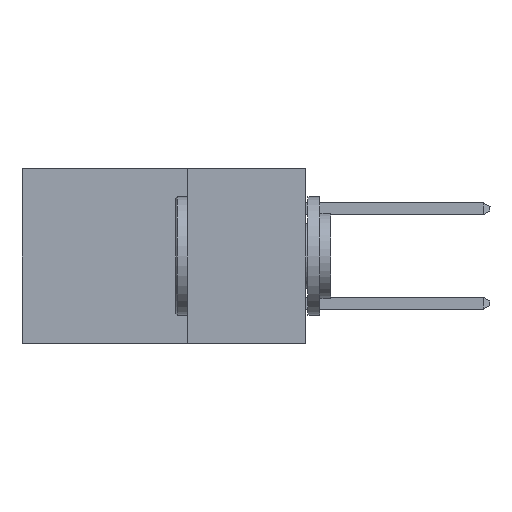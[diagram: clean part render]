
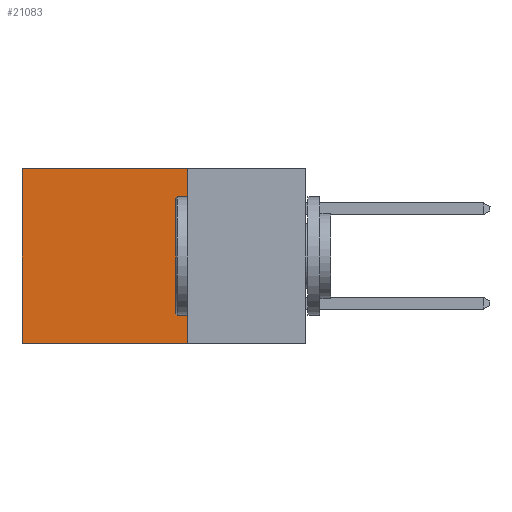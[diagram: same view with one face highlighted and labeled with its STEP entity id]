
A CAD part, left-side view. The second image highlights one B-rep face of the part: STEP entity #21083.
In plain terms, the highlighted planar face has unit normal (-1, 0, 0).
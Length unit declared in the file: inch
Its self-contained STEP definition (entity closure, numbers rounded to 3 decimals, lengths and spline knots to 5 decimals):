
#369 = CARTESIAN_POINT ( 'NONE',  ( 0.2615, 0.25, -0.37 ) ) ;
#415 = CARTESIAN_POINT ( 'NONE',  ( 0.2615, 0.6, 0. ) ) ;
#1843 = DIRECTION ( 'NONE',  ( 0., 0., -1. ) ) ;
#2372 = VECTOR ( 'NONE', #4687, 39.37008 ) ;
#2624 = EDGE_CURVE ( 'NONE', #24016, #11159, #25827, .T. ) ;
#3505 = FACE_OUTER_BOUND ( 'NONE', #10905, .T. ) ;
#4687 = DIRECTION ( 'NONE',  ( 0., 1., 0. ) ) ;
#6087 = PLANE ( 'NONE',  #12763 ) ;
#6592 = DIRECTION ( 'NONE',  ( 0., 0., -1. ) ) ;
#6895 = LINE ( 'NONE', #17288, #17645 ) ;
#8262 = CARTESIAN_POINT ( 'NONE',  ( 0.2615, 0.25, 0. ) ) ;
#8265 = DIRECTION ( 'NONE',  ( 1., 0., 0. ) ) ;
#8367 = CARTESIAN_POINT ( 'NONE',  ( 0.2615, 0.25, -0.37 ) ) ;
#8851 = ORIENTED_EDGE ( 'NONE', *, *, #27450, .F. ) ;
#9023 = LINE ( 'NONE', #8262, #25388 ) ;
#10343 = EDGE_CURVE ( 'NONE', #27089, #10607, #9023, .T. ) ;
#10457 = DIRECTION ( 'NONE',  ( 0., 1., 0. ) ) ;
#10607 = VERTEX_POINT ( 'NONE', #415 ) ;
#10905 = EDGE_LOOP ( 'NONE', ( #18181, #26465, #8851, #14825 ) ) ;
#11159 = VERTEX_POINT ( 'NONE', #25675 ) ;
#12477 = EDGE_CURVE ( 'NONE', #10607, #11159, #20475, .T. ) ;
#12763 = AXIS2_PLACEMENT_3D ( 'NONE', #18915, #8265, #23208 ) ;
#14825 = ORIENTED_EDGE ( 'NONE', *, *, #10343, .T. ) ;
#15517 = VECTOR ( 'NONE', #1843, 39.37008 ) ;
#17288 = CARTESIAN_POINT ( 'NONE',  ( 0.2615, 0.25, -0.37 ) ) ;
#17645 = VECTOR ( 'NONE', #6592, 39.37008 ) ;
#18181 = ORIENTED_EDGE ( 'NONE', *, *, #12477, .T. ) ;
#18915 = CARTESIAN_POINT ( 'NONE',  ( 0.2615, 0.25, -0.37 ) ) ;
#20475 = LINE ( 'NONE', #27463, #15517 ) ;
#21083 = ADVANCED_FACE ( 'NONE', ( #3505 ), #6087, .F. ) ;
#23208 = DIRECTION ( 'NONE',  ( 0., 0., -1. ) ) ;
#24016 = VERTEX_POINT ( 'NONE', #369 ) ;
#24364 = CARTESIAN_POINT ( 'NONE',  ( 0.2615, 0.25, 0. ) ) ;
#25388 = VECTOR ( 'NONE', #10457, 39.37008 ) ;
#25675 = CARTESIAN_POINT ( 'NONE',  ( 0.2615, 0.6, -0.37 ) ) ;
#25827 = LINE ( 'NONE', #8367, #2372 ) ;
#26465 = ORIENTED_EDGE ( 'NONE', *, *, #2624, .F. ) ;
#27089 = VERTEX_POINT ( 'NONE', #24364 ) ;
#27450 = EDGE_CURVE ( 'NONE', #27089, #24016, #6895, .T. ) ;
#27463 = CARTESIAN_POINT ( 'NONE',  ( 0.2615, 0.6, -0.37 ) ) ;
